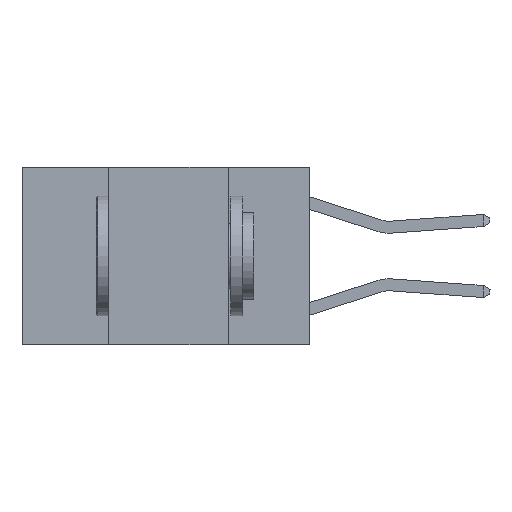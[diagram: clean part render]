
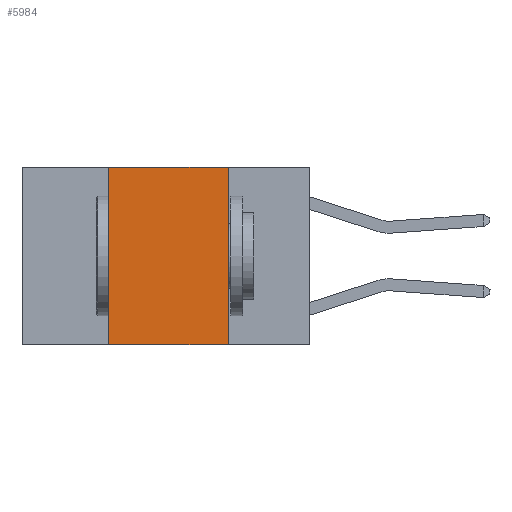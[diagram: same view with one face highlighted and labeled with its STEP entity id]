
A CAD part, left-side view. The second image highlights one B-rep face of the part: STEP entity #5984.
In plain terms, the highlighted planar face has unit normal (-1, 0, 0).
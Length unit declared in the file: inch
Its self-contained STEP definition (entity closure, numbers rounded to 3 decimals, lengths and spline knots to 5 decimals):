
#39 = CARTESIAN_POINT ( 'NONE',  ( 0., 0.42, -0.37 ) ) ;
#148 = DIRECTION ( 'NONE',  ( 0., 0., -1. ) ) ;
#271 = VECTOR ( 'NONE', #9101, 39.37008 ) ;
#537 = ORIENTED_EDGE ( 'NONE', *, *, #3405, .F. ) ;
#566 = CARTESIAN_POINT ( 'NONE',  ( 0., 0.42, 0. ) ) ;
#840 = LINE ( 'NONE', #9038, #271 ) ;
#934 = CARTESIAN_POINT ( 'NONE',  ( 0., 0.6, -0.37 ) ) ;
#1374 = CARTESIAN_POINT ( 'NONE',  ( 0., 0.17, 0. ) ) ;
#2565 = AXIS2_PLACEMENT_3D ( 'NONE', #2857, #5506, #148 ) ;
#2834 = CARTESIAN_POINT ( 'NONE',  ( 0., 0.42, 0. ) ) ;
#2857 = CARTESIAN_POINT ( 'NONE',  ( 0., 0.6, 0. ) ) ;
#3405 = EDGE_CURVE ( 'NONE', #6706, #9686, #4605, .T. ) ;
#4144 = EDGE_CURVE ( 'NONE', #9686, #10827, #840, .T. ) ;
#4587 = PLANE ( 'NONE',  #2565 ) ;
#4605 = LINE ( 'NONE', #6427, #10838 ) ;
#4737 = CARTESIAN_POINT ( 'NONE',  ( 0., 0.17, -0.37 ) ) ;
#4910 = DIRECTION ( 'NONE',  ( 0., -1., 0. ) ) ;
#4977 = VECTOR ( 'NONE', #8196, 39.37008 ) ;
#5279 = ORIENTED_EDGE ( 'NONE', *, *, #8441, .F. ) ;
#5506 = DIRECTION ( 'NONE',  ( 1., 0., 0. ) ) ;
#5984 = ADVANCED_FACE ( 'NONE', ( #8025 ), #4587, .F. ) ;
#6427 = CARTESIAN_POINT ( 'NONE',  ( 0., 0.6, 0. ) ) ;
#6706 = VERTEX_POINT ( 'NONE', #566 ) ;
#7470 = LINE ( 'NONE', #934, #4977 ) ;
#7471 = ORIENTED_EDGE ( 'NONE', *, *, #4144, .F. ) ;
#7647 = LINE ( 'NONE', #2834, #9611 ) ;
#7782 = ORIENTED_EDGE ( 'NONE', *, *, #9202, .T. ) ;
#8025 = FACE_OUTER_BOUND ( 'NONE', #8834, .T. ) ;
#8196 = DIRECTION ( 'NONE',  ( 0., -1., 0. ) ) ;
#8441 = EDGE_CURVE ( 'NONE', #11428, #6706, #7647, .T. ) ;
#8834 = EDGE_LOOP ( 'NONE', ( #7471, #537, #5279, #7782 ) ) ;
#9038 = CARTESIAN_POINT ( 'NONE',  ( 0., 0.17, 0. ) ) ;
#9073 = DIRECTION ( 'NONE',  ( 0., 0., 1. ) ) ;
#9101 = DIRECTION ( 'NONE',  ( 0., 0., -1. ) ) ;
#9202 = EDGE_CURVE ( 'NONE', #11428, #10827, #7470, .T. ) ;
#9611 = VECTOR ( 'NONE', #9073, 39.37008 ) ;
#9686 = VERTEX_POINT ( 'NONE', #1374 ) ;
#10827 = VERTEX_POINT ( 'NONE', #4737 ) ;
#10838 = VECTOR ( 'NONE', #4910, 39.37008 ) ;
#11428 = VERTEX_POINT ( 'NONE', #39 ) ;
